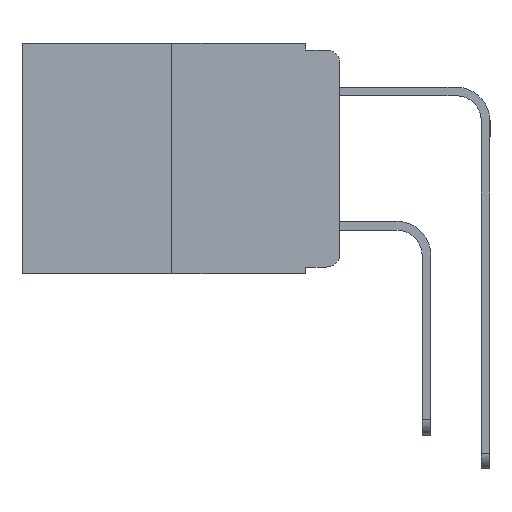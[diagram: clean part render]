
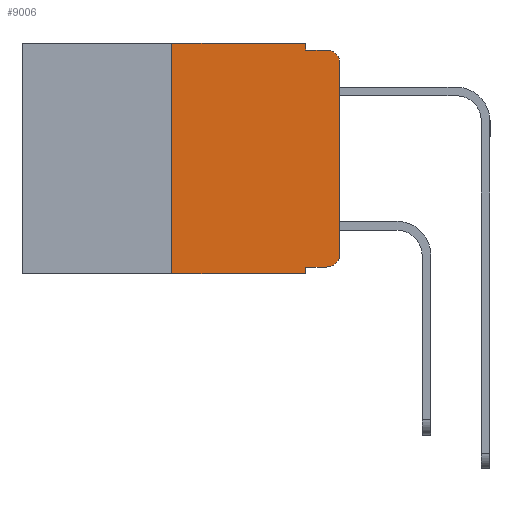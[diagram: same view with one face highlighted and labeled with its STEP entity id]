
A CAD part, left-side view. The second image highlights one B-rep face of the part: STEP entity #9006.
In plain terms, the highlighted planar face has unit normal (-1, 0, 0).
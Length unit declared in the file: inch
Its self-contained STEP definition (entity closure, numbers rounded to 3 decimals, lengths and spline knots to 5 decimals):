
#266 = DIRECTION ( 'NONE',  ( -1., 0., 0. ) ) ;
#270 = FACE_OUTER_BOUND ( 'NONE', #6345, .T. ) ;
#523 = CARTESIAN_POINT ( 'NONE',  ( 0., 0.25, 0. ) ) ;
#632 = CARTESIAN_POINT ( 'NONE',  ( 0., 0.473, 0. ) ) ;
#646 = VERTEX_POINT ( 'NONE', #7572 ) ;
#1533 = CARTESIAN_POINT ( 'NONE',  ( 0., 0.051, 0. ) ) ;
#1560 = DIRECTION ( 'NONE',  ( 0., 0., 1. ) ) ;
#1592 = CARTESIAN_POINT ( 'NONE',  ( 0., 0.051, -0.01 ) ) ;
#1731 = EDGE_CURVE ( 'NONE', #10860, #646, #8996, .T. ) ;
#1848 = DIRECTION ( 'NONE',  ( 0., 0., -1. ) ) ;
#1914 = LINE ( 'NONE', #12793, #6406 ) ;
#2448 = EDGE_CURVE ( 'NONE', #5473, #646, #11363, .T. ) ;
#2597 = CARTESIAN_POINT ( 'NONE',  ( 0., 0.051, -0.333 ) ) ;
#2733 = CARTESIAN_POINT ( 'NONE',  ( 0., 0.051, -0.343 ) ) ;
#2807 = LINE ( 'NONE', #2597, #5555 ) ;
#3117 = VERTEX_POINT ( 'NONE', #2733 ) ;
#3277 = CARTESIAN_POINT ( 'NONE',  ( 0., 0.051, -0.01 ) ) ;
#3351 = VERTEX_POINT ( 'NONE', #10071 ) ;
#3650 = DIRECTION ( 'NONE',  ( 0., -1., 0. ) ) ;
#3686 = VECTOR ( 'NONE', #13199, 39.37008 ) ;
#3747 = ORIENTED_EDGE ( 'NONE', *, *, #9424, .F. ) ;
#3904 = LINE ( 'NONE', #11518, #8777 ) ;
#4682 = DIRECTION ( 'NONE',  ( 0., -1., 0. ) ) ;
#4762 = ORIENTED_EDGE ( 'NONE', *, *, #5230, .T. ) ;
#4859 = ORIENTED_EDGE ( 'NONE', *, *, #12639, .F. ) ;
#5056 = LINE ( 'NONE', #1533, #10266 ) ;
#5159 = CARTESIAN_POINT ( 'NONE',  ( 0., 0.473, 0. ) ) ;
#5230 = EDGE_CURVE ( 'NONE', #9442, #5473, #1914, .T. ) ;
#5419 = CIRCLE ( 'NONE', #7884, 0.02 ) ;
#5473 = VERTEX_POINT ( 'NONE', #11847 ) ;
#5481 = VECTOR ( 'NONE', #1560, 39.37008 ) ;
#5555 = VECTOR ( 'NONE', #3650, 39.37008 ) ;
#5803 = LINE ( 'NONE', #9653, #5481 ) ;
#5831 = ORIENTED_EDGE ( 'NONE', *, *, #8791, .T. ) ;
#5921 = CARTESIAN_POINT ( 'NONE',  ( 0., 0.051, 0. ) ) ;
#6345 = EDGE_LOOP ( 'NONE', ( #4762, #10949, #9708, #4859, #10092, #12961, #10693, #3747, #5831, #6740 ) ) ;
#6406 = VECTOR ( 'NONE', #12844, 39.37008 ) ;
#6604 = VECTOR ( 'NONE', #10990, 39.37008 ) ;
#6659 = CARTESIAN_POINT ( 'NONE',  ( 0., 0.02, -0.313 ) ) ;
#6684 = VECTOR ( 'NONE', #6875, 39.37008 ) ;
#6740 = ORIENTED_EDGE ( 'NONE', *, *, #8166, .T. ) ;
#6875 = DIRECTION ( 'NONE',  ( 0., 0., -1. ) ) ;
#6925 = LINE ( 'NONE', #5159, #6604 ) ;
#6956 = PLANE ( 'NONE',  #7805 ) ;
#7327 = AXIS2_PLACEMENT_3D ( 'NONE', #10617, #11021, #9206 ) ;
#7572 = CARTESIAN_POINT ( 'NONE',  ( 0., 0.02, -0.01 ) ) ;
#7677 = DIRECTION ( 'NONE',  ( 0., 0., -1. ) ) ;
#7805 = AXIS2_PLACEMENT_3D ( 'NONE', #632, #7969, #1848 ) ;
#7884 = AXIS2_PLACEMENT_3D ( 'NONE', #6659, #266, #7677 ) ;
#7969 = DIRECTION ( 'NONE',  ( 1., 0., 0. ) ) ;
#7981 = CARTESIAN_POINT ( 'NONE',  ( 0., 0.051, -0.333 ) ) ;
#8166 = EDGE_CURVE ( 'NONE', #3351, #9442, #5419, .T. ) ;
#8205 = CARTESIAN_POINT ( 'NONE',  ( 0., 0.25, -0.343 ) ) ;
#8777 = VECTOR ( 'NONE', #4682, 39.37008 ) ;
#8791 = EDGE_CURVE ( 'NONE', #10439, #3351, #2807, .T. ) ;
#8938 = VERTEX_POINT ( 'NONE', #523 ) ;
#8996 = LINE ( 'NONE', #3277, #3686 ) ;
#9006 = ADVANCED_FACE ( 'NONE', ( #270 ), #6956, .F. ) ;
#9206 = DIRECTION ( 'NONE',  ( 0., 0., -1. ) ) ;
#9298 = LINE ( 'NONE', #9807, #6684 ) ;
#9424 = EDGE_CURVE ( 'NONE', #10439, #3117, #5056, .T. ) ;
#9442 = VERTEX_POINT ( 'NONE', #10585 ) ;
#9585 = DIRECTION ( 'NONE',  ( 0., 0., -1. ) ) ;
#9653 = CARTESIAN_POINT ( 'NONE',  ( 0., 0.25, 0. ) ) ;
#9708 = ORIENTED_EDGE ( 'NONE', *, *, #1731, .F. ) ;
#9752 = EDGE_CURVE ( 'NONE', #8938, #12670, #6925, .T. ) ;
#9807 = CARTESIAN_POINT ( 'NONE',  ( 0., 0.051, 0. ) ) ;
#10071 = CARTESIAN_POINT ( 'NONE',  ( 0., 0.02, -0.333 ) ) ;
#10092 = ORIENTED_EDGE ( 'NONE', *, *, #9752, .F. ) ;
#10230 = EDGE_CURVE ( 'NONE', #10566, #3117, #3904, .T. ) ;
#10266 = VECTOR ( 'NONE', #9585, 39.37008 ) ;
#10439 = VERTEX_POINT ( 'NONE', #7981 ) ;
#10566 = VERTEX_POINT ( 'NONE', #8205 ) ;
#10585 = CARTESIAN_POINT ( 'NONE',  ( 0., 0., -0.313 ) ) ;
#10617 = CARTESIAN_POINT ( 'NONE',  ( 0., 0.02, -0.03 ) ) ;
#10693 = ORIENTED_EDGE ( 'NONE', *, *, #10230, .T. ) ;
#10860 = VERTEX_POINT ( 'NONE', #1592 ) ;
#10949 = ORIENTED_EDGE ( 'NONE', *, *, #2448, .T. ) ;
#10990 = DIRECTION ( 'NONE',  ( 0., -1., 0. ) ) ;
#11021 = DIRECTION ( 'NONE',  ( -1., 0., 0. ) ) ;
#11363 = CIRCLE ( 'NONE', #7327, 0.02 ) ;
#11518 = CARTESIAN_POINT ( 'NONE',  ( 0., 0.473, -0.343 ) ) ;
#11847 = CARTESIAN_POINT ( 'NONE',  ( 0., 0., -0.03 ) ) ;
#11965 = EDGE_CURVE ( 'NONE', #10566, #8938, #5803, .T. ) ;
#12639 = EDGE_CURVE ( 'NONE', #12670, #10860, #9298, .T. ) ;
#12670 = VERTEX_POINT ( 'NONE', #5921 ) ;
#12793 = CARTESIAN_POINT ( 'NONE',  ( 0., 0., 0. ) ) ;
#12844 = DIRECTION ( 'NONE',  ( 0., 0., 1. ) ) ;
#12961 = ORIENTED_EDGE ( 'NONE', *, *, #11965, .F. ) ;
#13199 = DIRECTION ( 'NONE',  ( 0., -1., 0. ) ) ;
